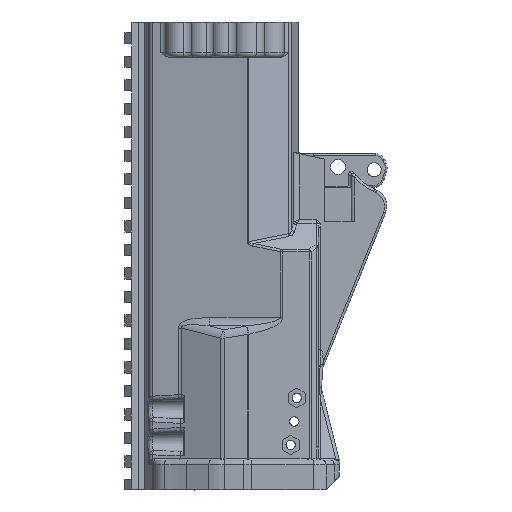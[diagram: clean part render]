
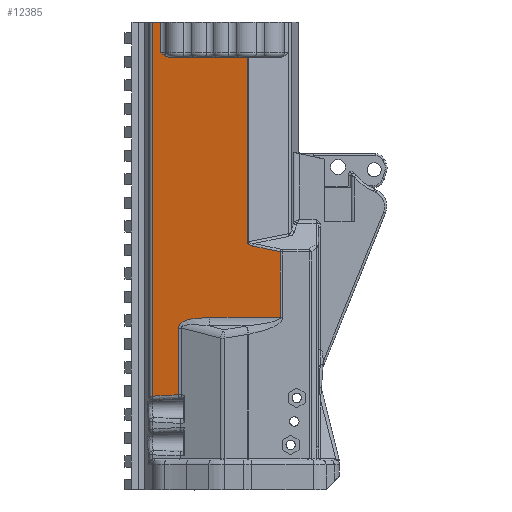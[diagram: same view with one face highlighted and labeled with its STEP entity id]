
A CAD part, left-side view. The second image highlights one B-rep face of the part: STEP entity #12385.
In plain terms, the highlighted planar face has unit normal (-0.979, 0.206, 0).
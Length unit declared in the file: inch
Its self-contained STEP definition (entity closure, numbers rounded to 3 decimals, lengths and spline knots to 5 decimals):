
#319=ELLIPSE('',#13382,1.75461,0.4);
#320=ELLIPSE('',#13383,0.31117,0.12);
#321=ELLIPSE('',#13384,1.14823,0.23622);
#559=B_SPLINE_CURVE_WITH_KNOTS('',3,(#23304,#23305,#23306,#23307,#23308,
#23309,#23310,#23311,#23312,#23313),.UNSPECIFIED.,.F.,.F.,(4,2,2,2,4),(-0.41537,
-0.33578,-0.2562,-0.1281,0.),
 .UNSPECIFIED.);
#756=PLANE('',#13381);
#1244=FACE_OUTER_BOUND('',#1971,.T.);
#1971=EDGE_LOOP('',(#9667,#9668,#9669,#9670,#9671,#9672,#9673,#9674,#9675,
#9676,#9677,#9678,#9679));
#2498=LINE('',#17793,#3492);
#2991=LINE('',#23283,#3985);
#2992=LINE('',#23288,#3986);
#2993=LINE('',#23292,#3987);
#2994=LINE('',#23294,#3988);
#2995=LINE('',#23296,#3989);
#2996=LINE('',#23300,#3990);
#2997=LINE('',#23302,#3991);
#2998=LINE('',#23314,#3992);
#3492=VECTOR('',#14238,0.3937);
#3985=VECTOR('',#15675,0.3937);
#3986=VECTOR('',#15680,0.3937);
#3987=VECTOR('',#15683,0.3937);
#3988=VECTOR('',#15684,0.3937);
#3989=VECTOR('',#15685,0.3937);
#3990=VECTOR('',#15688,0.3937);
#3991=VECTOR('',#15689,0.3937);
#3992=VECTOR('',#15690,0.3937);
#5033=VERTEX_POINT('',#17790);
#5034=VERTEX_POINT('',#17792);
#5768=VERTEX_POINT('',#23282);
#5769=VERTEX_POINT('',#23286);
#5770=VERTEX_POINT('',#23287);
#5771=VERTEX_POINT('',#23289);
#5772=VERTEX_POINT('',#23291);
#5773=VERTEX_POINT('',#23293);
#5774=VERTEX_POINT('',#23295);
#5775=VERTEX_POINT('',#23297);
#5776=VERTEX_POINT('',#23299);
#5777=VERTEX_POINT('',#23301);
#5778=VERTEX_POINT('',#23303);
#6256=EDGE_CURVE('',#5034,#5033,#2498,.T.);
#7221=EDGE_CURVE('',#5768,#5033,#2991,.T.);
#7223=EDGE_CURVE('',#5769,#5770,#2992,.T.);
#7224=EDGE_CURVE('',#5771,#5769,#319,.T.);
#7225=EDGE_CURVE('',#5772,#5771,#2993,.T.);
#7226=EDGE_CURVE('',#5773,#5772,#2994,.T.);
#7227=EDGE_CURVE('',#5774,#5773,#2995,.T.);
#7228=EDGE_CURVE('',#5775,#5774,#320,.T.);
#7229=EDGE_CURVE('',#5776,#5775,#2996,.T.);
#7230=EDGE_CURVE('',#5776,#5777,#2997,.T.);
#7231=EDGE_CURVE('',#5778,#5777,#559,.F.);
#7232=EDGE_CURVE('',#5034,#5778,#2998,.T.);
#7233=EDGE_CURVE('',#5770,#5768,#321,.T.);
#9667=ORIENTED_EDGE('',*,*,#7223,.F.);
#9668=ORIENTED_EDGE('',*,*,#7224,.F.);
#9669=ORIENTED_EDGE('',*,*,#7225,.F.);
#9670=ORIENTED_EDGE('',*,*,#7226,.F.);
#9671=ORIENTED_EDGE('',*,*,#7227,.F.);
#9672=ORIENTED_EDGE('',*,*,#7228,.F.);
#9673=ORIENTED_EDGE('',*,*,#7229,.F.);
#9674=ORIENTED_EDGE('',*,*,#7230,.T.);
#9675=ORIENTED_EDGE('',*,*,#7231,.F.);
#9676=ORIENTED_EDGE('',*,*,#7232,.F.);
#9677=ORIENTED_EDGE('',*,*,#6256,.T.);
#9678=ORIENTED_EDGE('',*,*,#7221,.F.);
#9679=ORIENTED_EDGE('',*,*,#7233,.F.);
#12385=ADVANCED_FACE('',(#1244),#756,.T.);
#13381=AXIS2_PLACEMENT_3D('',#23285,#15678,#15679);
#13382=AXIS2_PLACEMENT_3D('',#23290,#15681,#15682);
#13383=AXIS2_PLACEMENT_3D('',#23298,#15686,#15687);
#13384=AXIS2_PLACEMENT_3D('',#23315,#15691,#15692);
#14238=DIRECTION('',(0.206,0.979,0.));
#15675=DIRECTION('',(0.,0.,1.));
#15678=DIRECTION('center_axis',(-0.979,0.206,0.));
#15679=DIRECTION('ref_axis',(-0.206,-0.979,0.));
#15680=DIRECTION('',(0.,0.,-1.));
#15681=DIRECTION('center_axis',(-0.979,0.206,0.));
#15682=DIRECTION('ref_axis',(0.2,0.951,0.234));
#15683=DIRECTION('',(0.206,0.979,0.));
#15684=DIRECTION('',(0.,0.,-1.));
#15685=DIRECTION('',(-0.202,-0.959,-0.202));
#15686=DIRECTION('center_axis',(-0.979,0.206,0.));
#15687=DIRECTION('ref_axis',(0.201,0.957,-0.208));
#15688=DIRECTION('',(0.,0.,-1.));
#15689=DIRECTION('',(0.206,0.979,0.));
#15690=DIRECTION('',(0.,0.,-1.));
#15691=DIRECTION('center_axis',(-0.979,0.206,0.));
#15692=DIRECTION('ref_axis',(0.206,0.979,0.));
#17790=CARTESIAN_POINT('',(-0.73495,0.59981,5.49557));
#17792=CARTESIAN_POINT('',(-0.76358,0.46364,5.49557));
#17793=CARTESIAN_POINT('',(-0.88188,-0.09914,5.49557));
#23282=CARTESIAN_POINT('',(-0.73495,0.59981,-0.77254));
#23283=CARTESIAN_POINT('',(-0.73495,0.59981,-2.40157));
#23285=CARTESIAN_POINT('Origin',(-0.75194,0.51901,-2.40157));
#23286=CARTESIAN_POINT('',(-0.82661,0.16378,0.37061));
#23287=CARTESIAN_POINT('',(-0.82661,0.16378,-0.74982));
#23288=CARTESIAN_POINT('',(-0.82661,0.16378,-2.40157));
#23289=CARTESIAN_POINT('',(-0.93646,-0.35876,0.54741));
#23290=CARTESIAN_POINT('Origin',(-1.17808,-1.50808,-0.01828));
#23291=CARTESIAN_POINT('',(-1.18489,-1.5405,0.54741));
#23292=CARTESIAN_POINT('',(-0.80119,0.28469,0.54741));
#23293=CARTESIAN_POINT('',(-1.18489,-1.5405,1.64677));
#23294=CARTESIAN_POINT('',(-1.18489,-1.5405,-2.40157));
#23295=CARTESIAN_POINT('',(-1.08779,-1.0786,1.74387));
#23296=CARTESIAN_POINT('',(-1.07463,-1.016,1.75703));
#23297=CARTESIAN_POINT('',(-1.06853,-0.98699,1.81515));
#23298=CARTESIAN_POINT('Origin',(-1.13136,-1.28586,1.87001));
#23299=CARTESIAN_POINT('',(-1.06853,-0.98699,4.90502));
#23300=CARTESIAN_POINT('',(-1.06853,-0.98699,-2.40157));
#23301=CARTESIAN_POINT('',(-0.79501,0.31412,4.90502));
#23302=CARTESIAN_POINT('',(-0.8733,-0.05833,4.90502));
#23303=CARTESIAN_POINT('',(-0.76358,0.46364,4.98002));
#23304=CARTESIAN_POINT('Ctrl Pts',(-0.79501,0.31412,
4.90502));
#23305=CARTESIAN_POINT('Ctrl Pts',(-0.79286,0.32435,
4.90502));
#23306=CARTESIAN_POINT('Ctrl Pts',(-0.79053,0.33542,
4.90647));
#23307=CARTESIAN_POINT('Ctrl Pts',(-0.78599,0.357,
4.91197));
#23308=CARTESIAN_POINT('Ctrl Pts',(-0.78378,0.36752,
4.91598));
#23309=CARTESIAN_POINT('Ctrl Pts',(-0.77868,0.39178,
4.9273));
#23310=CARTESIAN_POINT('Ctrl Pts',(-0.77545,0.40717,
4.93682));
#23311=CARTESIAN_POINT('Ctrl Pts',(-0.76925,0.43663,
4.95799));
#23312=CARTESIAN_POINT('Ctrl Pts',(-0.76628,0.45077,
4.96954));
#23313=CARTESIAN_POINT('Ctrl Pts',(-0.76358,0.46364,
4.98002));
#23314=CARTESIAN_POINT('',(-0.76358,0.46364,5.49557));
#23315=CARTESIAN_POINT('Origin',(-0.83646,0.11696,-0.98583));
